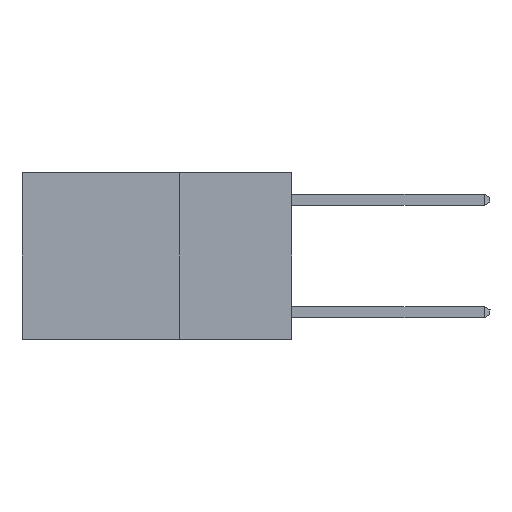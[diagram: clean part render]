
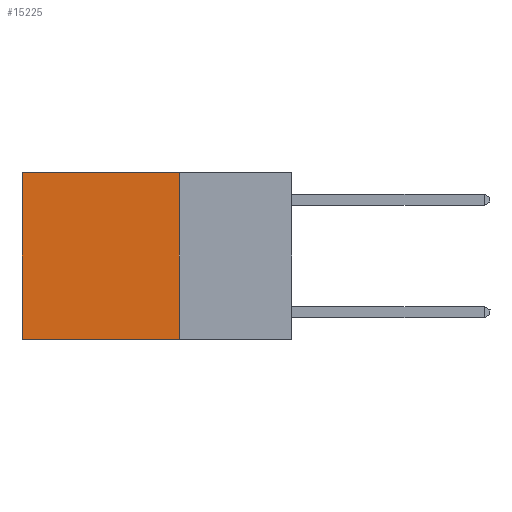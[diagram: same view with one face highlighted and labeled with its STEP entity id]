
A CAD part, left-side view. The second image highlights one B-rep face of the part: STEP entity #15225.
In plain terms, the highlighted planar face has unit normal (-1, 0, 0).
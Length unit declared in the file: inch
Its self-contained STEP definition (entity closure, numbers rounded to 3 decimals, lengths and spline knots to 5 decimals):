
#110 = PLANE ( 'NONE',  #4411 ) ;
#500 = EDGE_CURVE ( 'NONE', #3333, #11838, #3468, .T. ) ;
#3333 = VERTEX_POINT ( 'NONE', #15632 ) ;
#3468 = LINE ( 'NONE', #15079, #14872 ) ;
#3577 = ORIENTED_EDGE ( 'NONE', *, *, #12589, .F. ) ;
#4140 = EDGE_CURVE ( 'NONE', #10519, #15203, #13562, .T. ) ;
#4347 = VECTOR ( 'NONE', #16458, 39.37008 ) ;
#4411 = AXIS2_PLACEMENT_3D ( 'NONE', #7848, #6550, #7621 ) ;
#4997 = DIRECTION ( 'NONE',  ( 0., 1., 0. ) ) ;
#5762 = ORIENTED_EDGE ( 'NONE', *, *, #4140, .F. ) ;
#6230 = CARTESIAN_POINT ( 'NONE',  ( 0.2625, 0.25, 0. ) ) ;
#6550 = DIRECTION ( 'NONE',  ( 1., 0., 0. ) ) ;
#6779 = FACE_OUTER_BOUND ( 'NONE', #7525, .T. ) ;
#7525 = EDGE_LOOP ( 'NONE', ( #9458, #3577, #5762, #11115 ) ) ;
#7621 = DIRECTION ( 'NONE',  ( 0., 0., -1. ) ) ;
#7766 = CARTESIAN_POINT ( 'NONE',  ( 0.2625, 0.25, 0. ) ) ;
#7848 = CARTESIAN_POINT ( 'NONE',  ( 0.2625, 0.25, 0. ) ) ;
#8308 = VECTOR ( 'NONE', #4997, 39.37008 ) ;
#9458 = ORIENTED_EDGE ( 'NONE', *, *, #500, .T. ) ;
#9459 = VECTOR ( 'NONE', #12170, 39.37008 ) ;
#10271 = CARTESIAN_POINT ( 'NONE',  ( 0.2625, 0.25, 0. ) ) ;
#10519 = VERTEX_POINT ( 'NONE', #7766 ) ;
#10980 = EDGE_CURVE ( 'NONE', #10519, #3333, #11720, .T. ) ;
#11115 = ORIENTED_EDGE ( 'NONE', *, *, #10980, .T. ) ;
#11720 = LINE ( 'NONE', #10271, #8308 ) ;
#11838 = VERTEX_POINT ( 'NONE', #15733 ) ;
#12170 = DIRECTION ( 'NONE',  ( 0., 1., 0. ) ) ;
#12589 = EDGE_CURVE ( 'NONE', #15203, #11838, #14258, .T. ) ;
#13562 = LINE ( 'NONE', #6230, #4347 ) ;
#14258 = LINE ( 'NONE', #14539, #9459 ) ;
#14539 = CARTESIAN_POINT ( 'NONE',  ( 0.2625, 0.25, -0.37 ) ) ;
#14872 = VECTOR ( 'NONE', #16243, 39.37008 ) ;
#15079 = CARTESIAN_POINT ( 'NONE',  ( 0.2625, 0.6, 0. ) ) ;
#15203 = VERTEX_POINT ( 'NONE', #15514 ) ;
#15225 = ADVANCED_FACE ( 'NONE', ( #6779 ), #110, .F. ) ;
#15514 = CARTESIAN_POINT ( 'NONE',  ( 0.2625, 0.25, -0.37 ) ) ;
#15632 = CARTESIAN_POINT ( 'NONE',  ( 0.2625, 0.6, 0. ) ) ;
#15733 = CARTESIAN_POINT ( 'NONE',  ( 0.2625, 0.6, -0.37 ) ) ;
#16243 = DIRECTION ( 'NONE',  ( 0., 0., -1. ) ) ;
#16458 = DIRECTION ( 'NONE',  ( 0., 0., -1. ) ) ;
